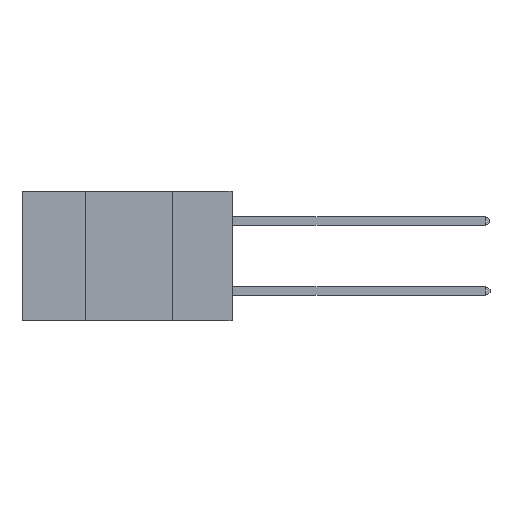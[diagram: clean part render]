
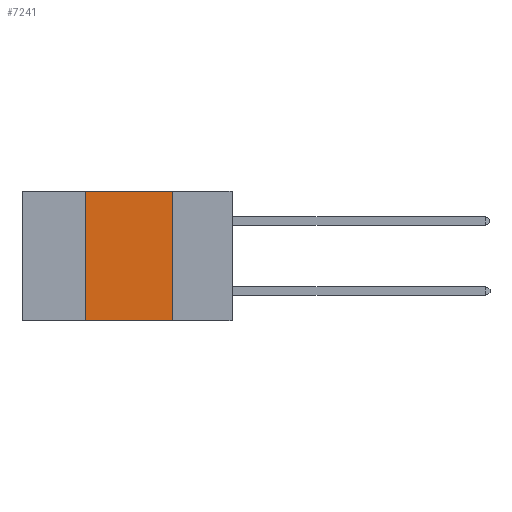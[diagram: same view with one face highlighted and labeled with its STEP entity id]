
A CAD part, left-side view. The second image highlights one B-rep face of the part: STEP entity #7241.
In plain terms, the highlighted planar face has unit normal (-1, 0, 0).
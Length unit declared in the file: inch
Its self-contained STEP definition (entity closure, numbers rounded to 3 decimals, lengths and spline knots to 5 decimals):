
#126 = CARTESIAN_POINT ( 'NONE',  ( 0., 0.6, 0. ) ) ;
#230 = PLANE ( 'NONE',  #8787 ) ;
#1071 = EDGE_LOOP ( 'NONE', ( #1934, #2067, #2493, #2841 ) ) ;
#1934 = ORIENTED_EDGE ( 'NONE', *, *, #9312, .F. ) ;
#2048 = DIRECTION ( 'NONE',  ( 0., 0., -1. ) ) ;
#2067 = ORIENTED_EDGE ( 'NONE', *, *, #5945, .F. ) ;
#2463 = CARTESIAN_POINT ( 'NONE',  ( 0., 0.17, 0. ) ) ;
#2493 = ORIENTED_EDGE ( 'NONE', *, *, #9493, .F. ) ;
#2841 = ORIENTED_EDGE ( 'NONE', *, *, #9256, .T. ) ;
#2903 = VERTEX_POINT ( 'NONE', #20470 ) ;
#4669 = CARTESIAN_POINT ( 'NONE',  ( 0., 0.42, 0. ) ) ;
#5945 = EDGE_CURVE ( 'NONE', #7854, #13926, #19803, .T. ) ;
#6164 = VECTOR ( 'NONE', #7749, 39.37008 ) ;
#7147 = DIRECTION ( 'NONE',  ( 0., -1., 0. ) ) ;
#7241 = ADVANCED_FACE ( 'NONE', ( #15510 ), #230, .F. ) ;
#7749 = DIRECTION ( 'NONE',  ( 0., 0., -1. ) ) ;
#7854 = VERTEX_POINT ( 'NONE', #20872 ) ;
#8787 = AXIS2_PLACEMENT_3D ( 'NONE', #20559, #12405, #2048 ) ;
#9256 = EDGE_CURVE ( 'NONE', #2903, #17686, #12336, .T. ) ;
#9312 = EDGE_CURVE ( 'NONE', #13926, #17686, #19538, .T. ) ;
#9493 = EDGE_CURVE ( 'NONE', #2903, #7854, #20269, .T. ) ;
#12336 = LINE ( 'NONE', #20802, #20525 ) ;
#12405 = DIRECTION ( 'NONE',  ( 1., 0., 0. ) ) ;
#12591 = VECTOR ( 'NONE', #16492, 39.37008 ) ;
#12660 = DIRECTION ( 'NONE',  ( 0., -1., 0. ) ) ;
#13926 = VERTEX_POINT ( 'NONE', #14795 ) ;
#14795 = CARTESIAN_POINT ( 'NONE',  ( 0., 0.17, 0. ) ) ;
#15415 = VECTOR ( 'NONE', #7147, 39.37008 ) ;
#15510 = FACE_OUTER_BOUND ( 'NONE', #1071, .T. ) ;
#16492 = DIRECTION ( 'NONE',  ( 0., 0., 1. ) ) ;
#17686 = VERTEX_POINT ( 'NONE', #19624 ) ;
#19538 = LINE ( 'NONE', #2463, #6164 ) ;
#19624 = CARTESIAN_POINT ( 'NONE',  ( 0., 0.17, -0.37 ) ) ;
#19803 = LINE ( 'NONE', #126, #15415 ) ;
#20269 = LINE ( 'NONE', #4669, #12591 ) ;
#20470 = CARTESIAN_POINT ( 'NONE',  ( 0., 0.42, -0.37 ) ) ;
#20525 = VECTOR ( 'NONE', #12660, 39.37008 ) ;
#20559 = CARTESIAN_POINT ( 'NONE',  ( 0., 0.6, 0. ) ) ;
#20802 = CARTESIAN_POINT ( 'NONE',  ( 0., 0.6, -0.37 ) ) ;
#20872 = CARTESIAN_POINT ( 'NONE',  ( 0., 0.42, 0. ) ) ;
